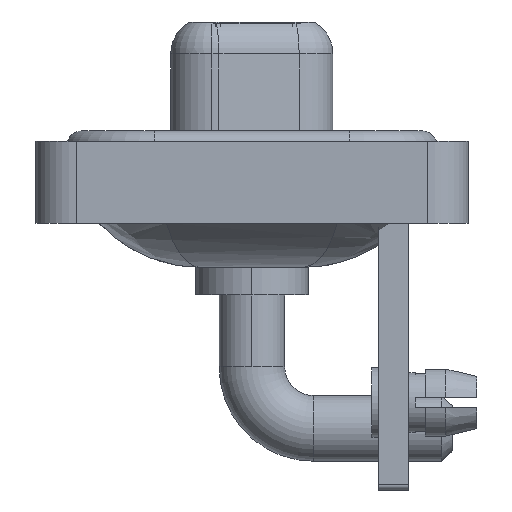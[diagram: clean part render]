
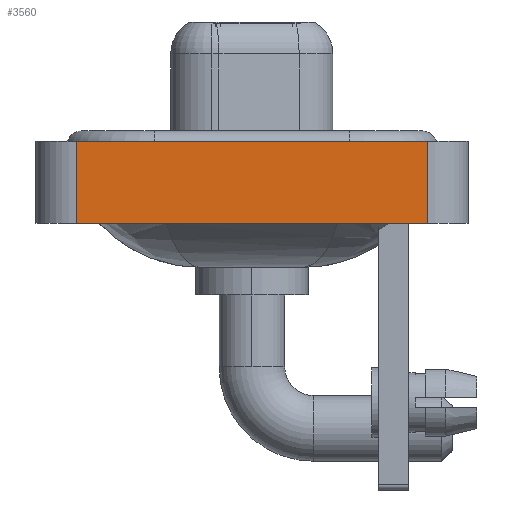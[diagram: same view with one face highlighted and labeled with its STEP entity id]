
A CAD part, left-side view. The second image highlights one B-rep face of the part: STEP entity #3560.
In plain terms, the highlighted planar face has unit normal (-1, 0, 0).
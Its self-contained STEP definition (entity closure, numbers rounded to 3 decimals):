
#109 = DIRECTION ( 'NONE',  ( -1., 0., 0. ) ) ;
#894 = VERTEX_POINT ( 'NONE', #18292 ) ;
#896 = DIRECTION ( 'NONE',  ( 0., 0., 1. ) ) ;
#1287 = LINE ( 'NONE', #11462, #5118 ) ;
#1672 = FACE_OUTER_BOUND ( 'NONE', #6294, .T. ) ;
#1810 = CARTESIAN_POINT ( 'NONE',  ( -7.35, -8.55, -3.6 ) ) ;
#2176 = CARTESIAN_POINT ( 'NONE',  ( -7.35, -8.55, 0.4 ) ) ;
#3560 = ADVANCED_FACE ( 'NONE', ( #1672 ), #15093, .T. ) ;
#3965 = AXIS2_PLACEMENT_3D ( 'NONE', #10599, #109, #16452 ) ;
#4254 = CARTESIAN_POINT ( 'NONE',  ( -7.35, 8.55, -3.6 ) ) ;
#5118 = VECTOR ( 'NONE', #15976, 1000. ) ;
#5917 = ORIENTED_EDGE ( 'NONE', *, *, #8443, .T. ) ;
#6152 = EDGE_CURVE ( 'NONE', #18186, #894, #13427, .T. ) ;
#6294 = EDGE_LOOP ( 'NONE', ( #5917, #8209, #18738, #11155 ) ) ;
#6852 = LINE ( 'NONE', #15374, #8273 ) ;
#6961 = CARTESIAN_POINT ( 'NONE',  ( -7.35, -8.55, -3.6 ) ) ;
#7681 = DIRECTION ( 'NONE',  ( 0., -1., 0. ) ) ;
#8209 = ORIENTED_EDGE ( 'NONE', *, *, #10942, .F. ) ;
#8273 = VECTOR ( 'NONE', #18450, 1000. ) ;
#8443 = EDGE_CURVE ( 'NONE', #894, #15006, #17117, .T. ) ;
#8566 = CARTESIAN_POINT ( 'NONE',  ( -7.35, 8.55, 0.4 ) ) ;
#10599 = CARTESIAN_POINT ( 'NONE',  ( -7.35, -8.55, -3.6 ) ) ;
#10942 = EDGE_CURVE ( 'NONE', #18121, #15006, #1287, .T. ) ;
#11155 = ORIENTED_EDGE ( 'NONE', *, *, #6152, .T. ) ;
#11462 = CARTESIAN_POINT ( 'NONE',  ( -7.35, -8.55, 0.4 ) ) ;
#12755 = VECTOR ( 'NONE', #896, 1000. ) ;
#13427 = LINE ( 'NONE', #1810, #15842 ) ;
#15006 = VERTEX_POINT ( 'NONE', #2176 ) ;
#15093 = PLANE ( 'NONE',  #3965 ) ;
#15374 = CARTESIAN_POINT ( 'NONE',  ( -7.35, 8.55, -3.6 ) ) ;
#15500 = EDGE_CURVE ( 'NONE', #18186, #18121, #6852, .T. ) ;
#15842 = VECTOR ( 'NONE', #7681, 1000. ) ;
#15976 = DIRECTION ( 'NONE',  ( 0., -1., 0. ) ) ;
#16452 = DIRECTION ( 'NONE',  ( 0., 0., 1. ) ) ;
#17117 = LINE ( 'NONE', #6961, #12755 ) ;
#18121 = VERTEX_POINT ( 'NONE', #8566 ) ;
#18186 = VERTEX_POINT ( 'NONE', #4254 ) ;
#18292 = CARTESIAN_POINT ( 'NONE',  ( -7.35, -8.55, -3.6 ) ) ;
#18450 = DIRECTION ( 'NONE',  ( 0., 0., 1. ) ) ;
#18738 = ORIENTED_EDGE ( 'NONE', *, *, #15500, .F. ) ;
